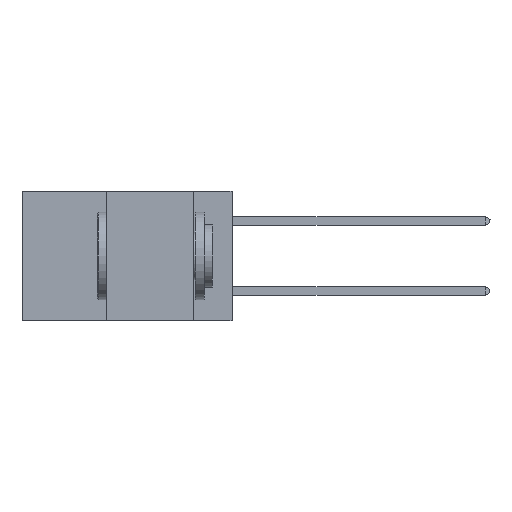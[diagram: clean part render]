
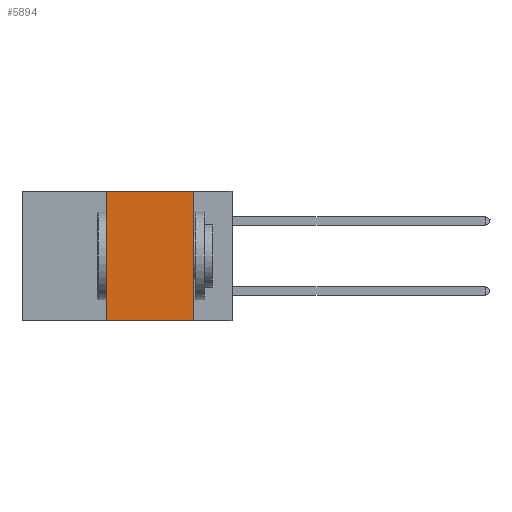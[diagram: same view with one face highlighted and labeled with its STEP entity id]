
A CAD part, left-side view. The second image highlights one B-rep face of the part: STEP entity #5894.
In plain terms, the highlighted planar face has unit normal (-1, 0, 0).
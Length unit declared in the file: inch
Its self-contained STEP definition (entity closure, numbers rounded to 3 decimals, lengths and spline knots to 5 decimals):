
#1176 = ORIENTED_EDGE ( 'NONE', *, *, #11965, .F. ) ;
#1720 = DIRECTION ( 'NONE',  ( 0., -1., 0. ) ) ;
#1768 = CARTESIAN_POINT ( 'NONE',  ( 0., 0.6, 0. ) ) ;
#1883 = DIRECTION ( 'NONE',  ( 0., -1., 0. ) ) ;
#2259 = VECTOR ( 'NONE', #1883, 39.37008 ) ;
#2970 = CARTESIAN_POINT ( 'NONE',  ( 0., 0.36, 0. ) ) ;
#3131 = VECTOR ( 'NONE', #1720, 39.37008 ) ;
#3849 = CARTESIAN_POINT ( 'NONE',  ( 0., 0.6, -0.37 ) ) ;
#4364 = EDGE_CURVE ( 'NONE', #10061, #7167, #10539, .T. ) ;
#4765 = CARTESIAN_POINT ( 'NONE',  ( 0., 0.11, 0. ) ) ;
#4905 = LINE ( 'NONE', #3849, #2259 ) ;
#5063 = DIRECTION ( 'NONE',  ( 0., 0., -1. ) ) ;
#5074 = DIRECTION ( 'NONE',  ( 1., 0., 0. ) ) ;
#5090 = PLANE ( 'NONE',  #5655 ) ;
#5103 = CARTESIAN_POINT ( 'NONE',  ( 0., 0.6, 0. ) ) ;
#5127 = FACE_OUTER_BOUND ( 'NONE', #6285, .T. ) ;
#5655 = AXIS2_PLACEMENT_3D ( 'NONE', #5103, #5074, #5063 ) ;
#5837 = LINE ( 'NONE', #11856, #8301 ) ;
#5894 = ADVANCED_FACE ( 'NONE', ( #5127 ), #5090, .F. ) ;
#5898 = CARTESIAN_POINT ( 'NONE',  ( 0., 0.11, 0. ) ) ;
#6285 = EDGE_LOOP ( 'NONE', ( #1176, #11196, #9159, #7077 ) ) ;
#6731 = DIRECTION ( 'NONE',  ( 0., 0., -1. ) ) ;
#7077 = ORIENTED_EDGE ( 'NONE', *, *, #12028, .T. ) ;
#7167 = VERTEX_POINT ( 'NONE', #5898 ) ;
#7642 = VERTEX_POINT ( 'NONE', #11914 ) ;
#8026 = VECTOR ( 'NONE', #6731, 39.37008 ) ;
#8301 = VECTOR ( 'NONE', #9234, 39.37008 ) ;
#8769 = EDGE_CURVE ( 'NONE', #7642, #10061, #5837, .T. ) ;
#9159 = ORIENTED_EDGE ( 'NONE', *, *, #8769, .F. ) ;
#9234 = DIRECTION ( 'NONE',  ( 0., 0., 1. ) ) ;
#9818 = CARTESIAN_POINT ( 'NONE',  ( 0., 0.11, -0.37 ) ) ;
#10061 = VERTEX_POINT ( 'NONE', #2970 ) ;
#10539 = LINE ( 'NONE', #1768, #3131 ) ;
#10592 = LINE ( 'NONE', #4765, #8026 ) ;
#11196 = ORIENTED_EDGE ( 'NONE', *, *, #4364, .F. ) ;
#11652 = VERTEX_POINT ( 'NONE', #9818 ) ;
#11856 = CARTESIAN_POINT ( 'NONE',  ( 0., 0.36, 0. ) ) ;
#11914 = CARTESIAN_POINT ( 'NONE',  ( 0., 0.36, -0.37 ) ) ;
#11965 = EDGE_CURVE ( 'NONE', #7167, #11652, #10592, .T. ) ;
#12028 = EDGE_CURVE ( 'NONE', #7642, #11652, #4905, .T. ) ;
